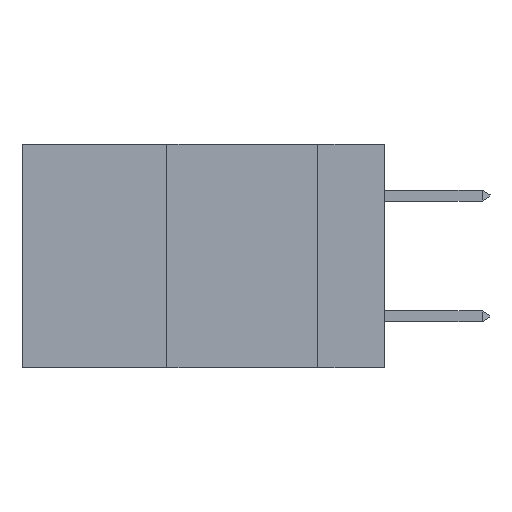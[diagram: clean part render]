
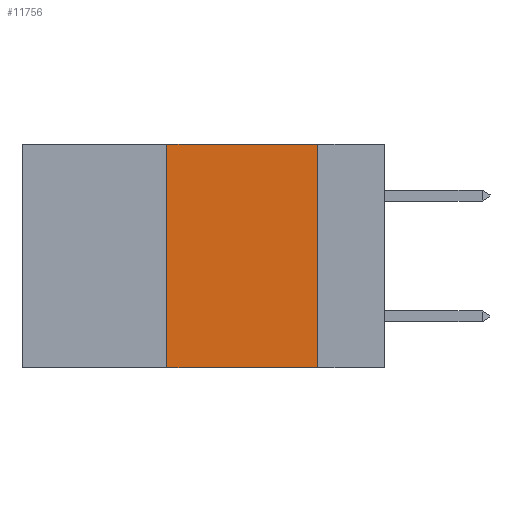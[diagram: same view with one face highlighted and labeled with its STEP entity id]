
A CAD part, left-side view. The second image highlights one B-rep face of the part: STEP entity #11756.
In plain terms, the highlighted planar face has unit normal (-1, 0, 0).
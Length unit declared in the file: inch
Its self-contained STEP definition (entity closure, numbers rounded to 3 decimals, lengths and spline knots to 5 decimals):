
#1498 = ORIENTED_EDGE ( 'NONE', *, *, #2510, .T. ) ;
#2510 = EDGE_CURVE ( 'NONE', #6586, #3557, #17664, .T. ) ;
#3131 = VECTOR ( 'NONE', #10144, 39.37008 ) ;
#3517 = DIRECTION ( 'NONE',  ( 0., 0., -1. ) ) ;
#3557 = VERTEX_POINT ( 'NONE', #5743 ) ;
#4044 = VECTOR ( 'NONE', #18662, 39.37008 ) ;
#4122 = ORIENTED_EDGE ( 'NONE', *, *, #6391, .F. ) ;
#4145 = CARTESIAN_POINT ( 'NONE',  ( 0., 0.6, 0. ) ) ;
#4167 = CARTESIAN_POINT ( 'NONE',  ( 0., 0.11, 0. ) ) ;
#4188 = CARTESIAN_POINT ( 'NONE',  ( 0., 0.36, -0.37 ) ) ;
#4338 = AXIS2_PLACEMENT_3D ( 'NONE', #10251, #16214, #10348 ) ;
#5193 = EDGE_CURVE ( 'NONE', #6586, #9962, #6709, .T. ) ;
#5317 = VERTEX_POINT ( 'NONE', #4167 ) ;
#5485 = ORIENTED_EDGE ( 'NONE', *, *, #5193, .F. ) ;
#5743 = CARTESIAN_POINT ( 'NONE',  ( 0., 0.11, -0.37 ) ) ;
#5763 = EDGE_CURVE ( 'NONE', #9962, #5317, #7072, .T. ) ;
#6391 = EDGE_CURVE ( 'NONE', #5317, #3557, #16933, .T. ) ;
#6586 = VERTEX_POINT ( 'NONE', #4188 ) ;
#6709 = LINE ( 'NONE', #17393, #4044 ) ;
#7072 = LINE ( 'NONE', #4145, #8480 ) ;
#8480 = VECTOR ( 'NONE', #10130, 39.37008 ) ;
#8996 = ORIENTED_EDGE ( 'NONE', *, *, #5763, .F. ) ;
#9962 = VERTEX_POINT ( 'NONE', #18710 ) ;
#10130 = DIRECTION ( 'NONE',  ( 0., -1., 0. ) ) ;
#10144 = DIRECTION ( 'NONE',  ( 0., -1., 0. ) ) ;
#10251 = CARTESIAN_POINT ( 'NONE',  ( 0., 0.6, 0. ) ) ;
#10348 = DIRECTION ( 'NONE',  ( 0., 0., -1. ) ) ;
#11624 = CARTESIAN_POINT ( 'NONE',  ( 0., 0.6, -0.37 ) ) ;
#11681 = VECTOR ( 'NONE', #3517, 39.37008 ) ;
#11756 = ADVANCED_FACE ( 'NONE', ( #11908 ), #19147, .F. ) ;
#11908 = FACE_OUTER_BOUND ( 'NONE', #13967, .T. ) ;
#13967 = EDGE_LOOP ( 'NONE', ( #4122, #8996, #5485, #1498 ) ) ;
#15548 = CARTESIAN_POINT ( 'NONE',  ( 0., 0.11, 0. ) ) ;
#16214 = DIRECTION ( 'NONE',  ( 1., 0., 0. ) ) ;
#16933 = LINE ( 'NONE', #15548, #11681 ) ;
#17393 = CARTESIAN_POINT ( 'NONE',  ( 0., 0.36, 0. ) ) ;
#17664 = LINE ( 'NONE', #11624, #3131 ) ;
#18662 = DIRECTION ( 'NONE',  ( 0., 0., 1. ) ) ;
#18710 = CARTESIAN_POINT ( 'NONE',  ( 0., 0.36, 0. ) ) ;
#19147 = PLANE ( 'NONE',  #4338 ) ;
